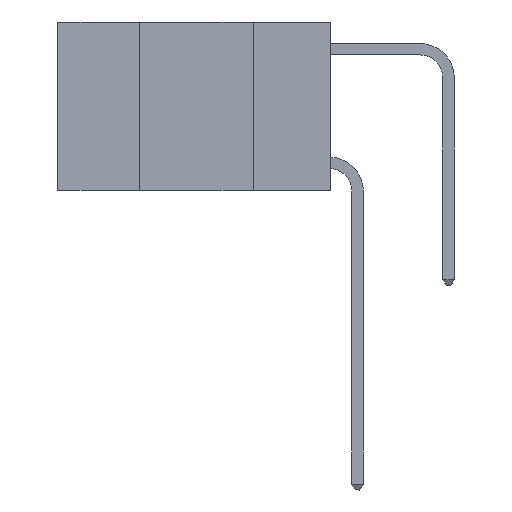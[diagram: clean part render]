
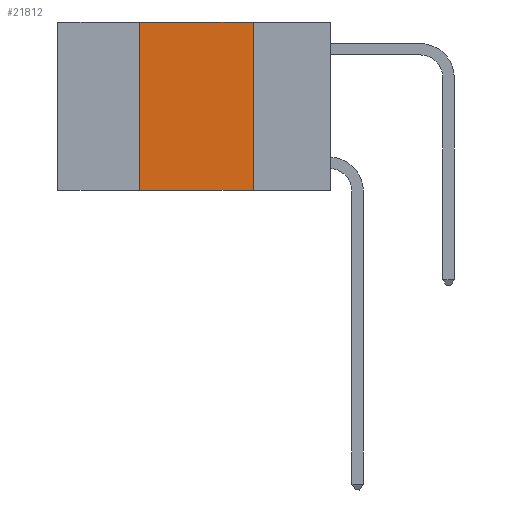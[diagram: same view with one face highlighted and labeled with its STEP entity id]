
A CAD part, left-side view. The second image highlights one B-rep face of the part: STEP entity #21812.
In plain terms, the highlighted planar face has unit normal (-1, 0, 0).
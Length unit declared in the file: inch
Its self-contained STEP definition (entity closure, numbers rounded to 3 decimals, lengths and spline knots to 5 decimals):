
#394 = EDGE_LOOP ( 'NONE', ( #13921, #18373, #22340, #8327 ) ) ;
#571 = DIRECTION ( 'NONE',  ( 0., -1., 0. ) ) ;
#748 = CARTESIAN_POINT ( 'NONE',  ( 0., 0.6, 0. ) ) ;
#1293 = LINE ( 'NONE', #14642, #10215 ) ;
#1594 = VERTEX_POINT ( 'NONE', #2266 ) ;
#2001 = EDGE_CURVE ( 'NONE', #20320, #1594, #2323, .T. ) ;
#2266 = CARTESIAN_POINT ( 'NONE',  ( 0., 0.17, -0.37 ) ) ;
#2323 = LINE ( 'NONE', #21165, #3788 ) ;
#2580 = EDGE_CURVE ( 'NONE', #16755, #13331, #1293, .T. ) ;
#2623 = VECTOR ( 'NONE', #10090, 39.37008 ) ;
#3788 = VECTOR ( 'NONE', #6076, 39.37008 ) ;
#3878 = EDGE_CURVE ( 'NONE', #16755, #1594, #21543, .T. ) ;
#4897 = DIRECTION ( 'NONE',  ( 0., 0., 1. ) ) ;
#5750 = CARTESIAN_POINT ( 'NONE',  ( 0., 0.42, 0. ) ) ;
#6076 = DIRECTION ( 'NONE',  ( 0., 0., -1. ) ) ;
#8327 = ORIENTED_EDGE ( 'NONE', *, *, #3878, .T. ) ;
#8370 = DIRECTION ( 'NONE',  ( 1., 0., 0. ) ) ;
#9710 = LINE ( 'NONE', #17259, #2623 ) ;
#9834 = CARTESIAN_POINT ( 'NONE',  ( 0., 0.42, -0.37 ) ) ;
#10090 = DIRECTION ( 'NONE',  ( 0., -1., 0. ) ) ;
#10215 = VECTOR ( 'NONE', #4897, 39.37008 ) ;
#10491 = PLANE ( 'NONE',  #11514 ) ;
#11514 = AXIS2_PLACEMENT_3D ( 'NONE', #748, #8370, #21837 ) ;
#12705 = EDGE_CURVE ( 'NONE', #13331, #20320, #9710, .T. ) ;
#13331 = VERTEX_POINT ( 'NONE', #5750 ) ;
#13921 = ORIENTED_EDGE ( 'NONE', *, *, #2001, .F. ) ;
#14097 = FACE_OUTER_BOUND ( 'NONE', #394, .T. ) ;
#14642 = CARTESIAN_POINT ( 'NONE',  ( 0., 0.42, 0. ) ) ;
#16755 = VERTEX_POINT ( 'NONE', #9834 ) ;
#17259 = CARTESIAN_POINT ( 'NONE',  ( 0., 0.6, 0. ) ) ;
#18373 = ORIENTED_EDGE ( 'NONE', *, *, #12705, .F. ) ;
#19381 = CARTESIAN_POINT ( 'NONE',  ( 0., 0.6, -0.37 ) ) ;
#20320 = VERTEX_POINT ( 'NONE', #22746 ) ;
#20899 = VECTOR ( 'NONE', #571, 39.37008 ) ;
#21165 = CARTESIAN_POINT ( 'NONE',  ( 0., 0.17, 0. ) ) ;
#21543 = LINE ( 'NONE', #19381, #20899 ) ;
#21812 = ADVANCED_FACE ( 'NONE', ( #14097 ), #10491, .F. ) ;
#21837 = DIRECTION ( 'NONE',  ( 0., 0., -1. ) ) ;
#22340 = ORIENTED_EDGE ( 'NONE', *, *, #2580, .F. ) ;
#22746 = CARTESIAN_POINT ( 'NONE',  ( 0., 0.17, 0. ) ) ;
